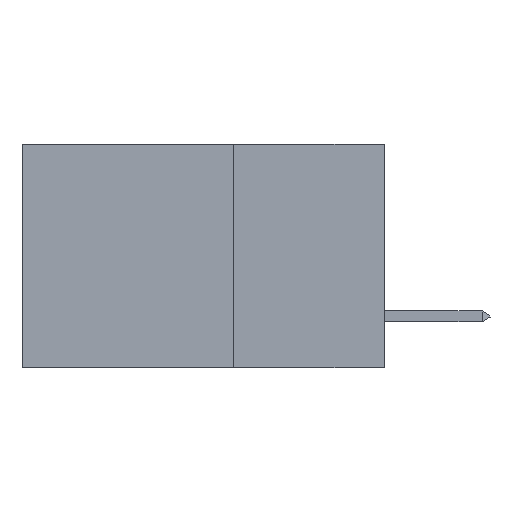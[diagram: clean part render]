
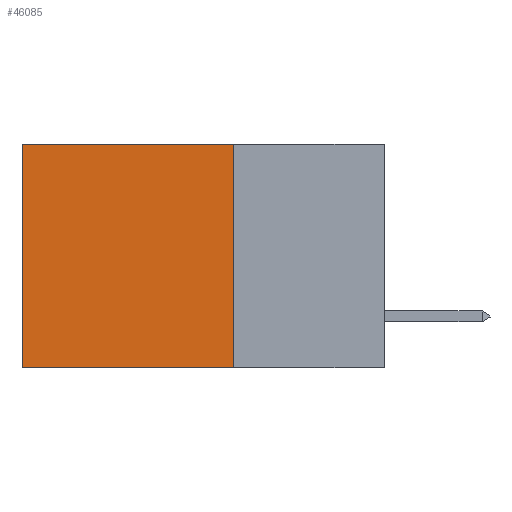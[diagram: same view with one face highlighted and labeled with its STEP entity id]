
A CAD part, left-side view. The second image highlights one B-rep face of the part: STEP entity #46085.
In plain terms, the highlighted planar face has unit normal (-1, 0, 0).
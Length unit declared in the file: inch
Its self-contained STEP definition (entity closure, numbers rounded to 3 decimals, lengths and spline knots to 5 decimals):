
#2505 = LINE ( 'NONE', #20112, #10903 ) ;
#2515 = AXIS2_PLACEMENT_3D ( 'NONE', #15789, #22986, #4206 ) ;
#2778 = CARTESIAN_POINT ( 'NONE',  ( 0.2875, 0.25, 0. ) ) ;
#4206 = DIRECTION ( 'NONE',  ( 0., 0., -1. ) ) ;
#6437 = VECTOR ( 'NONE', #44738, 39.37008 ) ;
#7630 = LINE ( 'NONE', #26126, #6437 ) ;
#8508 = CARTESIAN_POINT ( 'NONE',  ( 0.2875, 0.25, 0. ) ) ;
#8999 = FACE_OUTER_BOUND ( 'NONE', #14903, .T. ) ;
#10191 = CARTESIAN_POINT ( 'NONE',  ( 0.2875, 0.6, -0.37 ) ) ;
#10903 = VECTOR ( 'NONE', #44197, 39.37008 ) ;
#11023 = CARTESIAN_POINT ( 'NONE',  ( 0.2875, 0.25, -0.37 ) ) ;
#12639 = ORIENTED_EDGE ( 'NONE', *, *, #12874, .T. ) ;
#12874 = EDGE_CURVE ( 'NONE', #40849, #23269, #25593, .T. ) ;
#13953 = EDGE_CURVE ( 'NONE', #23269, #38669, #2505, .T. ) ;
#14903 = EDGE_LOOP ( 'NONE', ( #19632, #36454, #36927, #12639 ) ) ;
#15789 = CARTESIAN_POINT ( 'NONE',  ( 0.2875, 0.25, 0. ) ) ;
#19288 = LINE ( 'NONE', #8508, #25851 ) ;
#19632 = ORIENTED_EDGE ( 'NONE', *, *, #13953, .T. ) ;
#20112 = CARTESIAN_POINT ( 'NONE',  ( 0.2875, 0.6, 0. ) ) ;
#22981 = EDGE_CURVE ( 'NONE', #40849, #31162, #19288, .T. ) ;
#22986 = DIRECTION ( 'NONE',  ( 1., 0., 0. ) ) ;
#23269 = VERTEX_POINT ( 'NONE', #30602 ) ;
#24419 = VECTOR ( 'NONE', #48973, 39.37008 ) ;
#25593 = LINE ( 'NONE', #2778, #24419 ) ;
#25851 = VECTOR ( 'NONE', #47351, 39.37008 ) ;
#26126 = CARTESIAN_POINT ( 'NONE',  ( 0.2875, 0.25, -0.37 ) ) ;
#30602 = CARTESIAN_POINT ( 'NONE',  ( 0.2875, 0.6, 0. ) ) ;
#31162 = VERTEX_POINT ( 'NONE', #11023 ) ;
#32884 = CARTESIAN_POINT ( 'NONE',  ( 0.2875, 0.25, 0. ) ) ;
#34530 = PLANE ( 'NONE',  #2515 ) ;
#36454 = ORIENTED_EDGE ( 'NONE', *, *, #49197, .F. ) ;
#36927 = ORIENTED_EDGE ( 'NONE', *, *, #22981, .F. ) ;
#38669 = VERTEX_POINT ( 'NONE', #10191 ) ;
#40849 = VERTEX_POINT ( 'NONE', #32884 ) ;
#44197 = DIRECTION ( 'NONE',  ( 0., 0., -1. ) ) ;
#44738 = DIRECTION ( 'NONE',  ( 0., 1., 0. ) ) ;
#46085 = ADVANCED_FACE ( 'NONE', ( #8999 ), #34530, .F. ) ;
#47351 = DIRECTION ( 'NONE',  ( 0., 0., -1. ) ) ;
#48973 = DIRECTION ( 'NONE',  ( 0., 1., 0. ) ) ;
#49197 = EDGE_CURVE ( 'NONE', #31162, #38669, #7630, .T. ) ;
